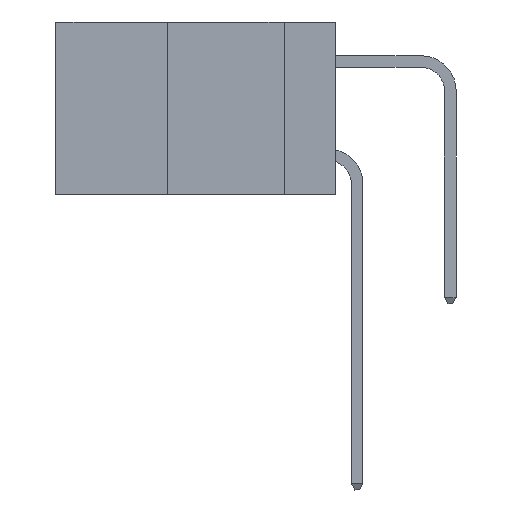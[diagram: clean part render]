
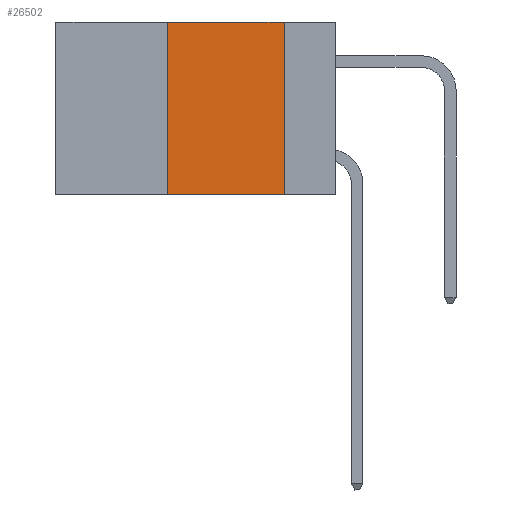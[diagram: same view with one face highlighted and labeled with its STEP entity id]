
A CAD part, left-side view. The second image highlights one B-rep face of the part: STEP entity #26502.
In plain terms, the highlighted planar face has unit normal (-1, 0, 0).
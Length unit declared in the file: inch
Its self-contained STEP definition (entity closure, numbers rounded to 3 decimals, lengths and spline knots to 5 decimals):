
#1 = LINE ( 'NONE', #3329, #23557 ) ;
#966 = VECTOR ( 'NONE', #20199, 39.37008 ) ;
#1417 = CARTESIAN_POINT ( 'NONE',  ( 0., 0.11, 0. ) ) ;
#2151 = CARTESIAN_POINT ( 'NONE',  ( 0., 0.36, 0. ) ) ;
#3329 = CARTESIAN_POINT ( 'NONE',  ( 0., 0.6, 0. ) ) ;
#4142 = DIRECTION ( 'NONE',  ( 0., 0., -1. ) ) ;
#4889 = AXIS2_PLACEMENT_3D ( 'NONE', #22955, #13599, #4142 ) ;
#5012 = CARTESIAN_POINT ( 'NONE',  ( 0., 0.11, -0.37 ) ) ;
#6109 = ORIENTED_EDGE ( 'NONE', *, *, #16620, .F. ) ;
#7938 = CARTESIAN_POINT ( 'NONE',  ( 0., 0.6, -0.37 ) ) ;
#7983 = EDGE_CURVE ( 'NONE', #12903, #23525, #1, .T. ) ;
#9398 = VERTEX_POINT ( 'NONE', #39632 ) ;
#12001 = EDGE_CURVE ( 'NONE', #9398, #28036, #20807, .T. ) ;
#12903 = VERTEX_POINT ( 'NONE', #2151 ) ;
#13599 = DIRECTION ( 'NONE',  ( 1., 0., 0. ) ) ;
#16620 = EDGE_CURVE ( 'NONE', #23525, #28036, #36830, .T. ) ;
#17872 = FACE_OUTER_BOUND ( 'NONE', #31750, .T. ) ;
#20199 = DIRECTION ( 'NONE',  ( 0., 0., -1. ) ) ;
#20807 = LINE ( 'NONE', #7938, #32113 ) ;
#21817 = EDGE_CURVE ( 'NONE', #9398, #12903, #33447, .T. ) ;
#21981 = DIRECTION ( 'NONE',  ( 0., -1., 0. ) ) ;
#22103 = DIRECTION ( 'NONE',  ( 0., 0., 1. ) ) ;
#22955 = CARTESIAN_POINT ( 'NONE',  ( 0., 0.6, 0. ) ) ;
#23491 = ORIENTED_EDGE ( 'NONE', *, *, #12001, .T. ) ;
#23525 = VERTEX_POINT ( 'NONE', #1417 ) ;
#23557 = VECTOR ( 'NONE', #21981, 39.37008 ) ;
#24567 = VECTOR ( 'NONE', #22103, 39.37008 ) ;
#25142 = CARTESIAN_POINT ( 'NONE',  ( 0., 0.36, 0. ) ) ;
#26260 = DIRECTION ( 'NONE',  ( 0., -1., 0. ) ) ;
#26502 = ADVANCED_FACE ( 'NONE', ( #17872 ), #38535, .F. ) ;
#28036 = VERTEX_POINT ( 'NONE', #5012 ) ;
#29399 = CARTESIAN_POINT ( 'NONE',  ( 0., 0.11, 0. ) ) ;
#31750 = EDGE_LOOP ( 'NONE', ( #6109, #39397, #32111, #23491 ) ) ;
#32111 = ORIENTED_EDGE ( 'NONE', *, *, #21817, .F. ) ;
#32113 = VECTOR ( 'NONE', #26260, 39.37008 ) ;
#33447 = LINE ( 'NONE', #25142, #24567 ) ;
#36830 = LINE ( 'NONE', #29399, #966 ) ;
#38535 = PLANE ( 'NONE',  #4889 ) ;
#39397 = ORIENTED_EDGE ( 'NONE', *, *, #7983, .F. ) ;
#39632 = CARTESIAN_POINT ( 'NONE',  ( 0., 0.36, -0.37 ) ) ;
